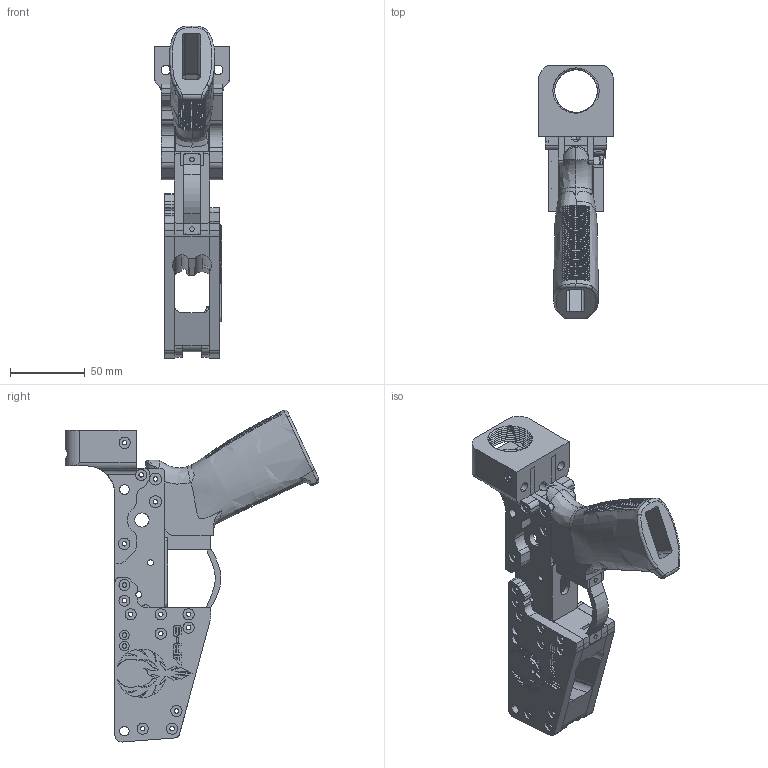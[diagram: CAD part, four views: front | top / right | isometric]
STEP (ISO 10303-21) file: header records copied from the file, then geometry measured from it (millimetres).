
FILE_DESCRIPTION (( 'STEP AP214' ), '1' );
FILE_NAME ('Firebolt_9_UBolt.STEP', '2020-12-05T18:47:57', ( '' ), ( '' ), 'SwSTEP 2.0', 'SolidWorks 2020', '' );
FILE_SCHEMA (( 'AUTOMOTIVE_DESIGN' ));
Length unit declared in the file: millimetre
Products named in the file (13): Mag_Release; Firebolt_9_UBolt; Firebolt_9_Mag_Well_Right; Firebolt_9_Mag_Well_Left; Firebolt_UBolt_Side_Right; Firebolt_Fire_Control_Well_Bottom; Firebolt_9_Mag_Well_Front; Firebolt_UBolt_Buffer_Tower; Firebolt_UBolt_Pistol_Grip; Firebolt_UBolt_Grip_Part; Firebolt_9_Mag_Well_Rear; Firebolt_UBolt_Side_Left; Firebolt_Trigger_Guard
Assembly tree (12 placements, depth 2):
  Firebolt_9_UBolt
    Firebolt_UBolt_Buffer_Tower
    Firebolt_UBolt_Side_Left
    Firebolt_UBolt_Side_Right
    Firebolt_UBolt_Grip_Part
    Firebolt_UBolt_Pistol_Grip
    Firebolt_Fire_Control_Well_Bottom
    Firebolt_Trigger_Guard
    Firebolt_9_Mag_Well_Rear
    Firebolt_9_Mag_Well_Right
    Firebolt_9_Mag_Well_Left
    Firebolt_9_Mag_Well_Front
    Mag_Release
Bounding box: 50 x 170.14 x 222.58 mm (x, y, z)
Volume: 293382 mm3; surface area: 127259.3 mm2
Topology: 12 solids, 12 shells, 2348 faces, 7069 edges, 4786 vertices
Faces by surface type: plane 1540, cylinder 501, bspline 277, cone 14, torus 9, sphere 7
Entity records: 145974 total; most frequent: CARTESIAN_POINT 85207, ORIENTED_EDGE 14128, DIRECTION 10252, EDGE_CURVE 7064, VERTEX_POINT 4786, LINE 4340, VECTOR 4340, AXIS2_PLACEMENT_3D 2956
